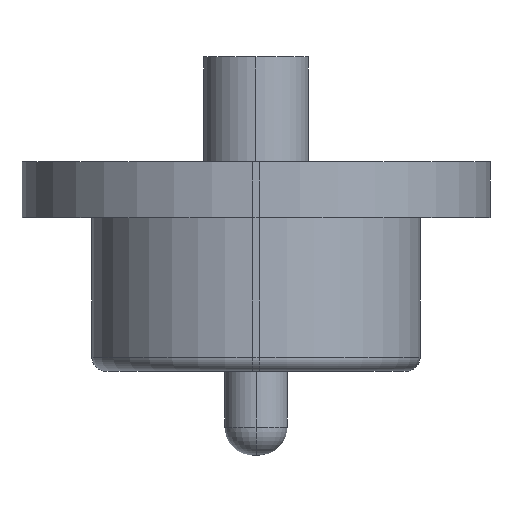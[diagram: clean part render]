
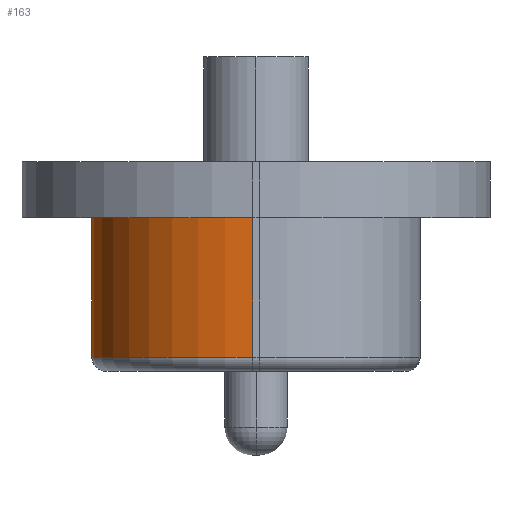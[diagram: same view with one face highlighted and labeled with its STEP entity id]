
A CAD part, left-side view. The second image highlights one B-rep face of the part: STEP entity #163.
In plain terms, the highlighted cylindrical face has radius 2.3 mm (diameter 4.6 mm), a partial arc.
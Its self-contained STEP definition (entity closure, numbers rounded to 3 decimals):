
#22 = VERTEX_POINT ( 'NONE', #4498 ) ;
#163 = ADVANCED_FACE ( 'NONE', ( #1728 ), #1398, .T. ) ;
#482 = EDGE_CURVE ( 'NONE', #3930, #4359, #5744, .T. ) ;
#963 = DIRECTION ( 'NONE',  ( 0., 0., -1. ) ) ;
#968 = CARTESIAN_POINT ( 'NONE',  ( -36.325, 15.05, 32.24 ) ) ;
#1140 = CARTESIAN_POINT ( 'NONE',  ( -36.325, 15.05, 30.4 ) ) ;
#1171 = DIRECTION ( 'NONE',  ( 0., 1., 0. ) ) ;
#1201 = EDGE_LOOP ( 'NONE', ( #3732, #1302, #3141, #5276 ) ) ;
#1302 = ORIENTED_EDGE ( 'NONE', *, *, #482, .T. ) ;
#1398 = CYLINDRICAL_SURFACE ( 'NONE', #3298, 2.3 ) ;
#1448 = AXIS2_PLACEMENT_3D ( 'NONE', #1140, #5634, #1171 ) ;
#1728 = FACE_OUTER_BOUND ( 'NONE', #1201, .T. ) ;
#1814 = VERTEX_POINT ( 'NONE', #2363 ) ;
#1910 = DIRECTION ( 'NONE',  ( 0., 0., -1. ) ) ;
#1991 = CARTESIAN_POINT ( 'NONE',  ( -36.325, 17.35, 30.2 ) ) ;
#2052 = LINE ( 'NONE', #1991, #3164 ) ;
#2363 = CARTESIAN_POINT ( 'NONE',  ( -38.625, 15.05, 30.4 ) ) ;
#2377 = EDGE_CURVE ( 'NONE', #22, #1814, #3785, .T. ) ;
#2878 = LINE ( 'NONE', #4642, #3961 ) ;
#3109 = DIRECTION ( 'NONE',  ( 0., -1., 0. ) ) ;
#3141 = ORIENTED_EDGE ( 'NONE', *, *, #4477, .F. ) ;
#3164 = VECTOR ( 'NONE', #3320, 1000. ) ;
#3298 = AXIS2_PLACEMENT_3D ( 'NONE', #968, #3968, #3109 ) ;
#3320 = DIRECTION ( 'NONE',  ( 0., 0., 1. ) ) ;
#3602 = AXIS2_PLACEMENT_3D ( 'NONE', #4540, #963, #5017 ) ;
#3732 = ORIENTED_EDGE ( 'NONE', *, *, #4331, .F. ) ;
#3785 = CIRCLE ( 'NONE', #1448, 2.3 ) ;
#3930 = VERTEX_POINT ( 'NONE', #4077 ) ;
#3961 = VECTOR ( 'NONE', #1910, 1000. ) ;
#3968 = DIRECTION ( 'NONE',  ( 0., 0., -1. ) ) ;
#4077 = CARTESIAN_POINT ( 'NONE',  ( -38.625, 15.05, 32.4 ) ) ;
#4331 = EDGE_CURVE ( 'NONE', #3930, #1814, #2878, .T. ) ;
#4359 = VERTEX_POINT ( 'NONE', #4455 ) ;
#4455 = CARTESIAN_POINT ( 'NONE',  ( -36.325, 17.35, 32.4 ) ) ;
#4477 = EDGE_CURVE ( 'NONE', #22, #4359, #2052, .T. ) ;
#4498 = CARTESIAN_POINT ( 'NONE',  ( -36.325, 17.35, 30.4 ) ) ;
#4540 = CARTESIAN_POINT ( 'NONE',  ( -36.325, 15.05, 32.4 ) ) ;
#4642 = CARTESIAN_POINT ( 'NONE',  ( -38.625, 15.05, 32.2 ) ) ;
#5017 = DIRECTION ( 'NONE',  ( -1., 0., 0. ) ) ;
#5276 = ORIENTED_EDGE ( 'NONE', *, *, #2377, .T. ) ;
#5634 = DIRECTION ( 'NONE',  ( 0., 0., 1. ) ) ;
#5744 = CIRCLE ( 'NONE', #3602, 2.3 ) ;
